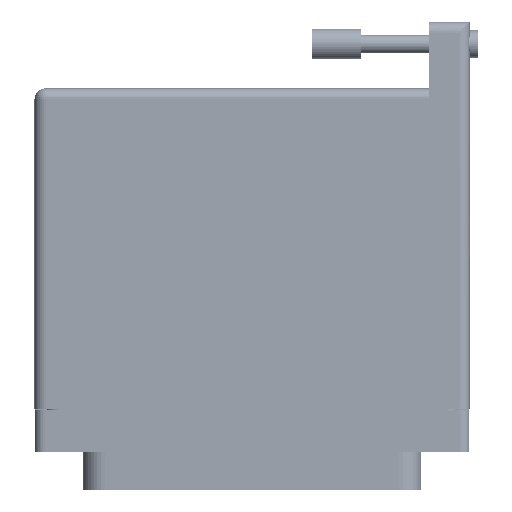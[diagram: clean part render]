
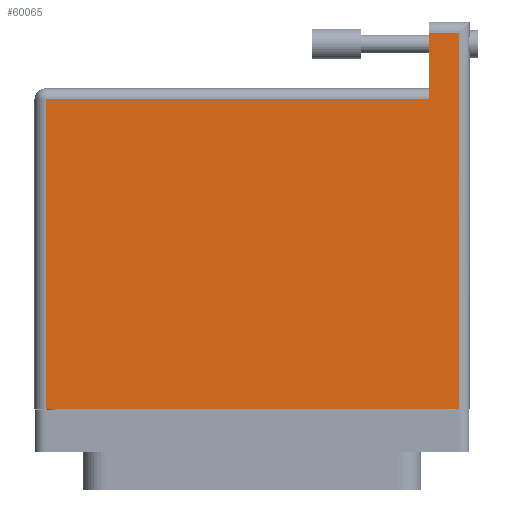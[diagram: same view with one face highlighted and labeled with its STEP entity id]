
A CAD part, front view. The second image highlights one B-rep face of the part: STEP entity #60065.
In plain terms, the highlighted face is planar.
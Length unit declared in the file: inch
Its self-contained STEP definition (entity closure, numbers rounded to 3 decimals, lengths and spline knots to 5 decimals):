
#3068 = LINE ( 'NONE', #8945, #25755 ) ;
#4430 = DIRECTION ( 'NONE',  ( 0., -1., 0. ) ) ;
#5674 = EDGE_CURVE ( 'NONE', #42239, #46317, #71086, .T. ) ;
#6702 = AXIS2_PLACEMENT_3D ( 'NONE', #34964, #84099, #83656 ) ;
#8078 = LINE ( 'NONE', #72417, #67733 ) ;
#8945 = CARTESIAN_POINT ( 'NONE',  ( -1.3775, 2.28, 0.765 ) ) ;
#11185 = CARTESIAN_POINT ( 'NONE',  ( 1.1215, 2.35, 0.765 ) ) ;
#13560 = DIRECTION ( 'NONE',  ( -1., 0., 0. ) ) ;
#14580 = VERTEX_POINT ( 'NONE', #84387 ) ;
#19557 = ORIENTED_EDGE ( 'NONE', *, *, #34253, .T. ) ;
#19876 = CARTESIAN_POINT ( 'NONE',  ( -1.3775, 1.86, 0.765 ) ) ;
#23733 = LINE ( 'NONE', #37703, #26866 ) ;
#24441 = VECTOR ( 'NONE', #69741, 39.37008 ) ;
#24898 = ORIENTED_EDGE ( 'NONE', *, *, #64688, .T. ) ;
#25755 = VECTOR ( 'NONE', #51784, 39.37008 ) ;
#26866 = VECTOR ( 'NONE', #85086, 39.37008 ) ;
#27312 = PLANE ( 'NONE',  #6702 ) ;
#28099 = ORIENTED_EDGE ( 'NONE', *, *, #58493, .T. ) ;
#34253 = EDGE_CURVE ( 'NONE', #61006, #81243, #72985, .T. ) ;
#34964 = CARTESIAN_POINT ( 'NONE',  ( -1.3775, 1.93, 0.765 ) ) ;
#35545 = VERTEX_POINT ( 'NONE', #65357 ) ;
#37703 = CARTESIAN_POINT ( 'NONE',  ( -1.3775, -0.1, 0.765 ) ) ;
#38079 = LINE ( 'NONE', #19876, #54908 ) ;
#41220 = EDGE_LOOP ( 'NONE', ( #19557, #24898, #73696, #28099, #55058, #74616 ) ) ;
#42033 = CARTESIAN_POINT ( 'NONE',  ( 1.1215, 1.86, 0.765 ) ) ;
#42239 = VERTEX_POINT ( 'NONE', #49817 ) ;
#46317 = VERTEX_POINT ( 'NONE', #67436 ) ;
#49142 = DIRECTION ( 'NONE',  ( 0., -1., 0. ) ) ;
#49470 = CARTESIAN_POINT ( 'NONE',  ( 1.3075, 2.35, 0.765 ) ) ;
#49817 = CARTESIAN_POINT ( 'NONE',  ( 1.3075, -0.1, 0.765 ) ) ;
#51784 = DIRECTION ( 'NONE',  ( -1., 0., 0. ) ) ;
#54908 = VECTOR ( 'NONE', #13560, 39.37008 ) ;
#55058 = ORIENTED_EDGE ( 'NONE', *, *, #5674, .T. ) ;
#56153 = FACE_OUTER_BOUND ( 'NONE', #41220, .T. ) ;
#58493 = EDGE_CURVE ( 'NONE', #35545, #42239, #23733, .T. ) ;
#59854 = VECTOR ( 'NONE', #4430, 39.37008 ) ;
#60065 = ADVANCED_FACE ( 'NONE', ( #56153 ), #27312, .F. ) ;
#61006 = VERTEX_POINT ( 'NONE', #79617 ) ;
#64688 = EDGE_CURVE ( 'NONE', #81243, #14580, #38079, .T. ) ;
#65357 = CARTESIAN_POINT ( 'NONE',  ( -1.3075, -0.1, 0.765 ) ) ;
#66458 = EDGE_CURVE ( 'NONE', #46317, #61006, #3068, .T. ) ;
#67436 = CARTESIAN_POINT ( 'NONE',  ( 1.3075, 2.28, 0.765 ) ) ;
#67733 = VECTOR ( 'NONE', #49142, 39.37008 ) ;
#68111 = EDGE_CURVE ( 'NONE', #14580, #35545, #8078, .T. ) ;
#69741 = DIRECTION ( 'NONE',  ( 0., 1., 0. ) ) ;
#71086 = LINE ( 'NONE', #49470, #24441 ) ;
#72417 = CARTESIAN_POINT ( 'NONE',  ( -1.3075, -0.1, 0.765 ) ) ;
#72985 = LINE ( 'NONE', #11185, #59854 ) ;
#73696 = ORIENTED_EDGE ( 'NONE', *, *, #68111, .T. ) ;
#74616 = ORIENTED_EDGE ( 'NONE', *, *, #66458, .T. ) ;
#79617 = CARTESIAN_POINT ( 'NONE',  ( 1.1215, 2.28, 0.765 ) ) ;
#81243 = VERTEX_POINT ( 'NONE', #42033 ) ;
#83656 = DIRECTION ( 'NONE',  ( -1., 0., 0. ) ) ;
#84099 = DIRECTION ( 'NONE',  ( 0., 0., -1. ) ) ;
#84387 = CARTESIAN_POINT ( 'NONE',  ( -1.3075, 1.86, 0.765 ) ) ;
#85086 = DIRECTION ( 'NONE',  ( 1., 0., 0. ) ) ;
